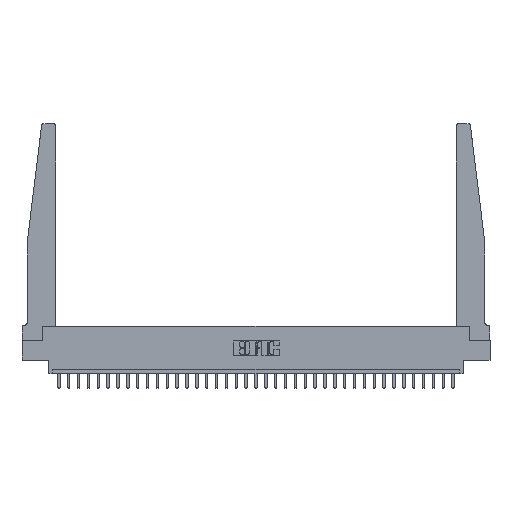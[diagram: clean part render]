
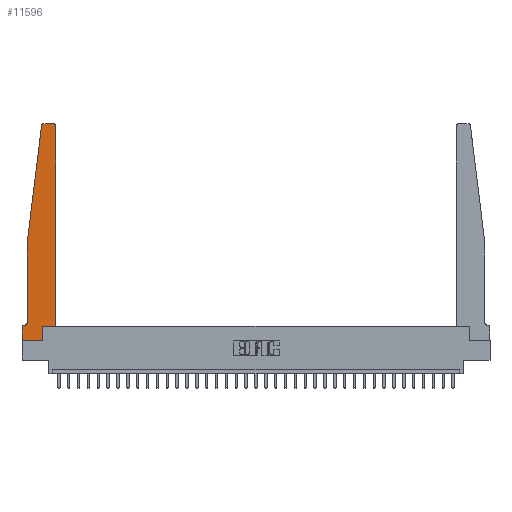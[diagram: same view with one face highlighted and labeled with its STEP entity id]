
A CAD part, top view. The second image highlights one B-rep face of the part: STEP entity #11596.
In plain terms, the highlighted planar face has unit normal (0, 0, 1).
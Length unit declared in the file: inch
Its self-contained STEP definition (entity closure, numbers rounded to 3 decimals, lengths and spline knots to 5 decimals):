
#272 = CARTESIAN_POINT ( 'NONE',  ( 0., 0.1875, 0.37 ) ) ;
#599 = EDGE_CURVE ( 'NONE', #1699, #27862, #20024, .T. ) ;
#1074 = EDGE_CURVE ( 'NONE', #1661, #16889, #11060, .T. ) ;
#1384 = DIRECTION ( 'NONE',  ( 0., 1., 0. ) ) ;
#1639 = AXIS2_PLACEMENT_3D ( 'NONE', #18254, #13045, #5718 ) ;
#1661 = VERTEX_POINT ( 'NONE', #14255 ) ;
#1699 = VERTEX_POINT ( 'NONE', #24456 ) ;
#1787 = CARTESIAN_POINT ( 'NONE',  ( 0.395, 2.72, 0.37 ) ) ;
#1964 = DIRECTION ( 'NONE',  ( 0., -1., 0. ) ) ;
#1998 = DIRECTION ( 'NONE',  ( 0., 1., 0. ) ) ;
#3184 = CARTESIAN_POINT ( 'NONE',  ( 0.2605, 0., 0.37 ) ) ;
#3232 = VERTEX_POINT ( 'NONE', #18204 ) ;
#3281 = VECTOR ( 'NONE', #1964, 39.37008 ) ;
#3308 = EDGE_CURVE ( 'NONE', #15075, #19517, #20854, .T. ) ;
#4024 = CARTESIAN_POINT ( 'NONE',  ( 0.395, 2.75, 0.37 ) ) ;
#4124 = VECTOR ( 'NONE', #30139, 39.37008 ) ;
#4410 = VECTOR ( 'NONE', #11273, 39.37008 ) ;
#4630 = AXIS2_PLACEMENT_3D ( 'NONE', #1787, #30043, #29883 ) ;
#5084 = VECTOR ( 'NONE', #1384, 39.37008 ) ;
#5182 = DIRECTION ( 'NONE',  ( 0., 0., 1. ) ) ;
#5552 = CARTESIAN_POINT ( 'NONE',  ( 0.425, 0.18, 0.37 ) ) ;
#5594 = AXIS2_PLACEMENT_3D ( 'NONE', #28432, #9586, #11465 ) ;
#5663 = EDGE_CURVE ( 'NONE', #15119, #9386, #28619, .T. ) ;
#5718 = DIRECTION ( 'NONE',  ( 1., 0., 0. ) ) ;
#5769 = FACE_OUTER_BOUND ( 'NONE', #28368, .T. ) ;
#6118 = VECTOR ( 'NONE', #17114, 39.37008 ) ;
#6349 = ORIENTED_EDGE ( 'NONE', *, *, #22761, .T. ) ;
#6490 = EDGE_CURVE ( 'NONE', #23465, #15119, #12004, .T. ) ;
#6723 = ORIENTED_EDGE ( 'NONE', *, *, #5663, .T. ) ;
#7517 = VERTEX_POINT ( 'NONE', #29364 ) ;
#7631 = CARTESIAN_POINT ( 'NONE',  ( 0.2605, 0.18, 0.37 ) ) ;
#8568 = EDGE_CURVE ( 'NONE', #16889, #24332, #30769, .T. ) ;
#8788 = EDGE_CURVE ( 'NONE', #9386, #1661, #17703, .T. ) ;
#9249 = CARTESIAN_POINT ( 'NONE',  ( 0.25, 2.75, 0.37 ) ) ;
#9386 = VERTEX_POINT ( 'NONE', #5552 ) ;
#9542 = ORIENTED_EDGE ( 'NONE', *, *, #14761, .T. ) ;
#9586 = DIRECTION ( 'NONE',  ( 0., 0., -1. ) ) ;
#9675 = DIRECTION ( 'NONE',  ( 1., 0., 0. ) ) ;
#9845 = DIRECTION ( 'NONE',  ( 1., 0., 0. ) ) ;
#11060 = CIRCLE ( 'NONE', #4630, 0.03 ) ;
#11200 = LINE ( 'NONE', #20781, #3281 ) ;
#11273 = DIRECTION ( 'NONE',  ( -0.122, -0.992, 0. ) ) ;
#11465 = DIRECTION ( 'NONE',  ( -1., 0., 0. ) ) ;
#11548 = ORIENTED_EDGE ( 'NONE', *, *, #6490, .T. ) ;
#11596 = ADVANCED_FACE ( 'NONE', ( #5769 ), #24891, .T. ) ;
#12004 = LINE ( 'NONE', #30396, #19926 ) ;
#13045 = DIRECTION ( 'NONE',  ( 0., 0., 1. ) ) ;
#13155 = CARTESIAN_POINT ( 'NONE',  ( 0.24675, 2.72367, 0.37 ) ) ;
#13541 = VECTOR ( 'NONE', #17686, 39.37008 ) ;
#13647 = CIRCLE ( 'NONE', #1639, 0.03 ) ;
#13754 = CARTESIAN_POINT ( 'NONE',  ( 0., 0.1875, 0.37 ) ) ;
#14255 = CARTESIAN_POINT ( 'NONE',  ( 0.425, 2.72, 0.37 ) ) ;
#14761 = EDGE_CURVE ( 'NONE', #3232, #1699, #30636, .T. ) ;
#15017 = EDGE_CURVE ( 'NONE', #19517, #3232, #22739, .T. ) ;
#15075 = VERTEX_POINT ( 'NONE', #13155 ) ;
#15119 = VERTEX_POINT ( 'NONE', #7631 ) ;
#15850 = CARTESIAN_POINT ( 'NONE',  ( 0.065, 1.25, 0.37 ) ) ;
#16889 = VERTEX_POINT ( 'NONE', #4024 ) ;
#17114 = DIRECTION ( 'NONE',  ( -1., 0., 0. ) ) ;
#17628 = ORIENTED_EDGE ( 'NONE', *, *, #15017, .T. ) ;
#17686 = DIRECTION ( 'NONE',  ( -1., 0., 0. ) ) ;
#17703 = LINE ( 'NONE', #30259, #5084 ) ;
#17776 = CARTESIAN_POINT ( 'NONE',  ( 0.065, 1.25, 0.37 ) ) ;
#17818 = EDGE_CURVE ( 'NONE', #7517, #23465, #28833, .T. ) ;
#18149 = ORIENTED_EDGE ( 'NONE', *, *, #8788, .T. ) ;
#18204 = CARTESIAN_POINT ( 'NONE',  ( 0.065, 0.2375, 0.37 ) ) ;
#18254 = CARTESIAN_POINT ( 'NONE',  ( 0.27653, 2.72, 0.37 ) ) ;
#19060 = ORIENTED_EDGE ( 'NONE', *, *, #8568, .T. ) ;
#19402 = CARTESIAN_POINT ( 'NONE',  ( 0., 0., 0.37 ) ) ;
#19517 = VERTEX_POINT ( 'NONE', #17776 ) ;
#19926 = VECTOR ( 'NONE', #1998, 39.37008 ) ;
#20024 = LINE ( 'NONE', #21921, #13541 ) ;
#20781 = CARTESIAN_POINT ( 'NONE',  ( 0., 0., 0.37 ) ) ;
#20854 = LINE ( 'NONE', #28079, #4410 ) ;
#21458 = ORIENTED_EDGE ( 'NONE', *, *, #30240, .T. ) ;
#21544 = CARTESIAN_POINT ( 'NONE',  ( 0.425, 0.18, 0.37 ) ) ;
#21921 = CARTESIAN_POINT ( 'NONE',  ( 0.065, 0.1875, 0.37 ) ) ;
#22490 = AXIS2_PLACEMENT_3D ( 'NONE', #272, #5182, #9845 ) ;
#22739 = LINE ( 'NONE', #15850, #4124 ) ;
#22761 = EDGE_CURVE ( 'NONE', #27862, #7517, #11200, .T. ) ;
#23465 = VERTEX_POINT ( 'NONE', #3184 ) ;
#24332 = VERTEX_POINT ( 'NONE', #30675 ) ;
#24406 = ORIENTED_EDGE ( 'NONE', *, *, #1074, .T. ) ;
#24456 = CARTESIAN_POINT ( 'NONE',  ( 0.015, 0.1875, 0.37 ) ) ;
#24891 = PLANE ( 'NONE',  #22490 ) ;
#24939 = DIRECTION ( 'NONE',  ( 1., 0., 0. ) ) ;
#27280 = VECTOR ( 'NONE', #24939, 39.37008 ) ;
#27774 = ORIENTED_EDGE ( 'NONE', *, *, #599, .T. ) ;
#27862 = VERTEX_POINT ( 'NONE', #13754 ) ;
#28079 = CARTESIAN_POINT ( 'NONE',  ( 0.065, 1.25, 0.37 ) ) ;
#28368 = EDGE_LOOP ( 'NONE', ( #19060, #21458, #29662, #17628, #9542, #27774, #6349, #30618, #11548, #6723, #18149, #24406 ) ) ;
#28432 = CARTESIAN_POINT ( 'NONE',  ( 0.015, 0.2375, 0.37 ) ) ;
#28619 = LINE ( 'NONE', #21544, #27280 ) ;
#28833 = LINE ( 'NONE', #19402, #30349 ) ;
#29364 = CARTESIAN_POINT ( 'NONE',  ( 0., 0., 0.37 ) ) ;
#29662 = ORIENTED_EDGE ( 'NONE', *, *, #3308, .T. ) ;
#29883 = DIRECTION ( 'NONE',  ( 1., 0., 0. ) ) ;
#30043 = DIRECTION ( 'NONE',  ( 0., 0., 1. ) ) ;
#30139 = DIRECTION ( 'NONE',  ( 0., -1., 0. ) ) ;
#30240 = EDGE_CURVE ( 'NONE', #24332, #15075, #13647, .T. ) ;
#30259 = CARTESIAN_POINT ( 'NONE',  ( 0.425, 0.18, 0.37 ) ) ;
#30349 = VECTOR ( 'NONE', #9675, 39.37008 ) ;
#30396 = CARTESIAN_POINT ( 'NONE',  ( 0.2605, 0.18, 0.37 ) ) ;
#30618 = ORIENTED_EDGE ( 'NONE', *, *, #17818, .T. ) ;
#30636 = CIRCLE ( 'NONE', #5594, 0.05 ) ;
#30675 = CARTESIAN_POINT ( 'NONE',  ( 0.27653, 2.75, 0.37 ) ) ;
#30769 = LINE ( 'NONE', #9249, #6118 ) ;
